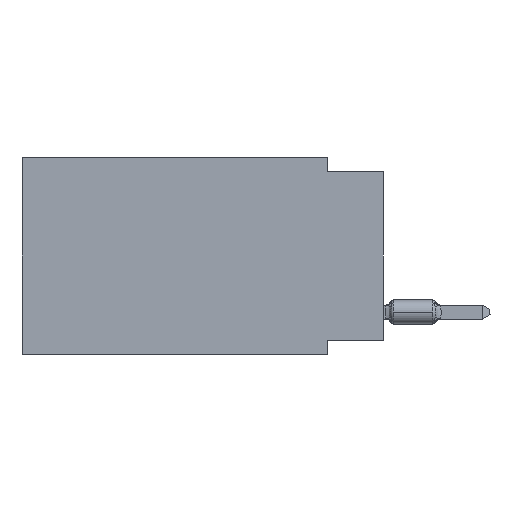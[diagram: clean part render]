
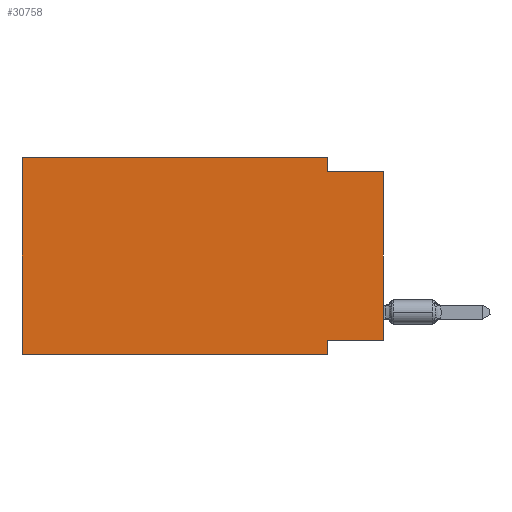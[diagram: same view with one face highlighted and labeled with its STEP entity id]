
A CAD part, left-side view. The second image highlights one B-rep face of the part: STEP entity #30758.
In plain terms, the highlighted planar face has unit normal (-1, 0, 0).
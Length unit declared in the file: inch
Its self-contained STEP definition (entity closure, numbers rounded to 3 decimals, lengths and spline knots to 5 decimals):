
#275 = ORIENTED_EDGE ( 'NONE', *, *, #18921, .F. ) ;
#1303 = CARTESIAN_POINT ( 'NONE',  ( 0., 0.1, -0.35 ) ) ;
#1381 = VECTOR ( 'NONE', #29302, 39.37008 ) ;
#4044 = CARTESIAN_POINT ( 'NONE',  ( 0., 0.645, 0. ) ) ;
#4264 = CARTESIAN_POINT ( 'NONE',  ( 0., 0.645, -0.35 ) ) ;
#4337 = DIRECTION ( 'NONE',  ( 0., 0., -1. ) ) ;
#4678 = CARTESIAN_POINT ( 'NONE',  ( 0., 0.1, 0. ) ) ;
#4834 = EDGE_CURVE ( 'NONE', #24909, #19808, #22468, .T. ) ;
#6446 = DIRECTION ( 'NONE',  ( 0., 0., 1. ) ) ;
#6950 = ORIENTED_EDGE ( 'NONE', *, *, #23822, .F. ) ;
#6983 = LINE ( 'NONE', #1303, #33293 ) ;
#9377 = FACE_OUTER_BOUND ( 'NONE', #25057, .T. ) ;
#9465 = DIRECTION ( 'NONE',  ( 0., -1., 0. ) ) ;
#9565 = DIRECTION ( 'NONE',  ( 0., 0., -1. ) ) ;
#10322 = EDGE_CURVE ( 'NONE', #13627, #17523, #32716, .T. ) ;
#10537 = CARTESIAN_POINT ( 'NONE',  ( 0., 0.1, 0. ) ) ;
#11083 = LINE ( 'NONE', #22107, #16873 ) ;
#11731 = DIRECTION ( 'NONE',  ( 0., -1., 0. ) ) ;
#12374 = DIRECTION ( 'NONE',  ( 0., 1., 0. ) ) ;
#13081 = VERTEX_POINT ( 'NONE', #34002 ) ;
#13627 = VERTEX_POINT ( 'NONE', #4264 ) ;
#13991 = ORIENTED_EDGE ( 'NONE', *, *, #10322, .T. ) ;
#14223 = CARTESIAN_POINT ( 'NONE',  ( 0., 0.1, -0.325 ) ) ;
#14507 = EDGE_CURVE ( 'NONE', #33222, #23961, #11083, .T. ) ;
#14770 = CARTESIAN_POINT ( 'NONE',  ( 0., 0., -0.325 ) ) ;
#15995 = VERTEX_POINT ( 'NONE', #14223 ) ;
#16873 = VECTOR ( 'NONE', #9465, 39.37008 ) ;
#17504 = CARTESIAN_POINT ( 'NONE',  ( 0., 0.1, -0.35 ) ) ;
#17521 = CARTESIAN_POINT ( 'NONE',  ( 0., 0., -0.325 ) ) ;
#17523 = VERTEX_POINT ( 'NONE', #17504 ) ;
#17980 = EDGE_CURVE ( 'NONE', #13081, #19808, #34464, .T. ) ;
#18371 = PLANE ( 'NONE',  #21921 ) ;
#18921 = EDGE_CURVE ( 'NONE', #13627, #33222, #35087, .T. ) ;
#18961 = VECTOR ( 'NONE', #12374, 39.37008 ) ;
#19101 = CARTESIAN_POINT ( 'NONE',  ( 0., 0., -0.025 ) ) ;
#19721 = ORIENTED_EDGE ( 'NONE', *, *, #26910, .F. ) ;
#19808 = VERTEX_POINT ( 'NONE', #19101 ) ;
#20155 = EDGE_CURVE ( 'NONE', #23961, #13081, #31180, .T. ) ;
#20824 = ORIENTED_EDGE ( 'NONE', *, *, #20155, .F. ) ;
#21751 = CARTESIAN_POINT ( 'NONE',  ( 0., 0.645, 0. ) ) ;
#21900 = VECTOR ( 'NONE', #22271, 39.37008 ) ;
#21921 = AXIS2_PLACEMENT_3D ( 'NONE', #4044, #31893, #9565 ) ;
#22107 = CARTESIAN_POINT ( 'NONE',  ( 0., 0.645, 0. ) ) ;
#22271 = DIRECTION ( 'NONE',  ( 0., 0., 1. ) ) ;
#22468 = LINE ( 'NONE', #34023, #35139 ) ;
#22791 = ORIENTED_EDGE ( 'NONE', *, *, #14507, .F. ) ;
#22854 = LINE ( 'NONE', #17521, #18961 ) ;
#23518 = VECTOR ( 'NONE', #11731, 39.37008 ) ;
#23822 = EDGE_CURVE ( 'NONE', #15995, #17523, #6983, .T. ) ;
#23961 = VERTEX_POINT ( 'NONE', #10537 ) ;
#24343 = CARTESIAN_POINT ( 'NONE',  ( 0., 0., -0.025 ) ) ;
#24909 = VERTEX_POINT ( 'NONE', #14770 ) ;
#25057 = EDGE_LOOP ( 'NONE', ( #26872, #27395, #20824, #22791, #275, #13991, #6950, #19721 ) ) ;
#25079 = CARTESIAN_POINT ( 'NONE',  ( 0., 0.645, 0. ) ) ;
#25239 = CARTESIAN_POINT ( 'NONE',  ( 0., 0.645, -0.35 ) ) ;
#26872 = ORIENTED_EDGE ( 'NONE', *, *, #4834, .T. ) ;
#26910 = EDGE_CURVE ( 'NONE', #24909, #15995, #22854, .T. ) ;
#27395 = ORIENTED_EDGE ( 'NONE', *, *, #17980, .F. ) ;
#29302 = DIRECTION ( 'NONE',  ( 0., -1., 0. ) ) ;
#30758 = ADVANCED_FACE ( 'NONE', ( #9377 ), #18371, .F. ) ;
#31180 = LINE ( 'NONE', #4678, #34981 ) ;
#31893 = DIRECTION ( 'NONE',  ( 1., 0., 0. ) ) ;
#32716 = LINE ( 'NONE', #25239, #23518 ) ;
#33222 = VERTEX_POINT ( 'NONE', #25079 ) ;
#33293 = VECTOR ( 'NONE', #4337, 39.37008 ) ;
#34002 = CARTESIAN_POINT ( 'NONE',  ( 0., 0.1, -0.025 ) ) ;
#34020 = DIRECTION ( 'NONE',  ( 0., 0., -1. ) ) ;
#34023 = CARTESIAN_POINT ( 'NONE',  ( 0., 0., 0. ) ) ;
#34464 = LINE ( 'NONE', #24343, #1381 ) ;
#34981 = VECTOR ( 'NONE', #34020, 39.37008 ) ;
#35087 = LINE ( 'NONE', #21751, #21900 ) ;
#35139 = VECTOR ( 'NONE', #6446, 39.37008 ) ;
